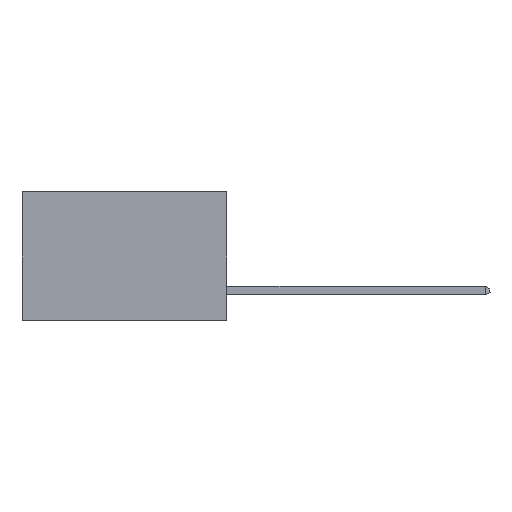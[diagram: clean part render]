
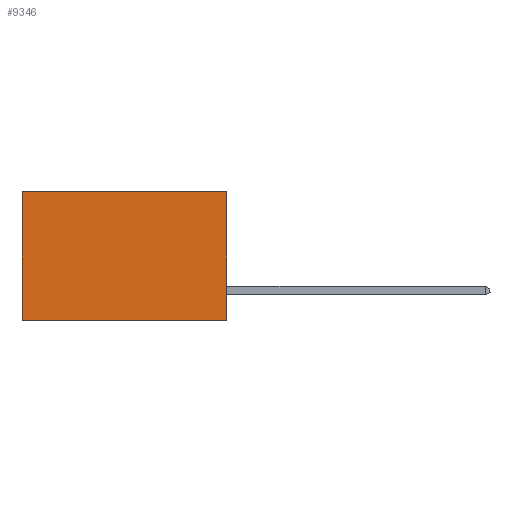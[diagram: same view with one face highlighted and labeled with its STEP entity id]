
A CAD part, left-side view. The second image highlights one B-rep face of the part: STEP entity #9346.
In plain terms, the highlighted planar face has unit normal (-1, 0, 0).
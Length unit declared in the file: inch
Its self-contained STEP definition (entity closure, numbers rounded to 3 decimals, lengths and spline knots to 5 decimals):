
#121 = EDGE_LOOP ( 'NONE', ( #21535, #1404, #6696, #2013 ) ) ;
#1185 = DIRECTION ( 'NONE',  ( 0., 0., -1. ) ) ;
#1189 = DIRECTION ( 'NONE',  ( 1., 0., 0. ) ) ;
#1210 = CARTESIAN_POINT ( 'NONE',  ( 0.277, 0., -0.37 ) ) ;
#1312 = EDGE_CURVE ( 'NONE', #15598, #20218, #22398, .T. ) ;
#1326 = PLANE ( 'NONE',  #8657 ) ;
#1404 = ORIENTED_EDGE ( 'NONE', *, *, #19868, .F. ) ;
#2013 = ORIENTED_EDGE ( 'NONE', *, *, #7317, .T. ) ;
#2120 = CARTESIAN_POINT ( 'NONE',  ( 0.277, 0.59, -0.37 ) ) ;
#2456 = VECTOR ( 'NONE', #13844, 39.37008 ) ;
#4245 = DIRECTION ( 'NONE',  ( 0., 0., -1. ) ) ;
#5901 = CARTESIAN_POINT ( 'NONE',  ( 0.277, 0.59, -0.37 ) ) ;
#6696 = ORIENTED_EDGE ( 'NONE', *, *, #8898, .F. ) ;
#6921 = CARTESIAN_POINT ( 'NONE',  ( 0.277, 0.59, 0. ) ) ;
#7317 = EDGE_CURVE ( 'NONE', #20247, #15598, #17886, .T. ) ;
#8657 = AXIS2_PLACEMENT_3D ( 'NONE', #1210, #1189, #1185 ) ;
#8898 = EDGE_CURVE ( 'NONE', #20247, #12622, #16341, .T. ) ;
#8998 = CARTESIAN_POINT ( 'NONE',  ( 0.277, 0., -0.37 ) ) ;
#9346 = ADVANCED_FACE ( 'NONE', ( #24883 ), #1326, .F. ) ;
#11001 = DIRECTION ( 'NONE',  ( 0., 1., 0. ) ) ;
#12545 = CARTESIAN_POINT ( 'NONE',  ( 0.277, 0., -0.37 ) ) ;
#12622 = VERTEX_POINT ( 'NONE', #12545 ) ;
#12802 = VECTOR ( 'NONE', #14337, 39.37008 ) ;
#13844 = DIRECTION ( 'NONE',  ( 0., 0., -1. ) ) ;
#14337 = DIRECTION ( 'NONE',  ( 0., 1., 0. ) ) ;
#14369 = CARTESIAN_POINT ( 'NONE',  ( 0.277, 0., 0. ) ) ;
#14669 = CARTESIAN_POINT ( 'NONE',  ( 0.277, 0., -0.37 ) ) ;
#15598 = VERTEX_POINT ( 'NONE', #6921 ) ;
#16341 = LINE ( 'NONE', #14669, #2456 ) ;
#17392 = VECTOR ( 'NONE', #4245, 39.37008 ) ;
#17886 = LINE ( 'NONE', #14369, #12802 ) ;
#19868 = EDGE_CURVE ( 'NONE', #12622, #20218, #20036, .T. ) ;
#20036 = LINE ( 'NONE', #8998, #24479 ) ;
#20218 = VERTEX_POINT ( 'NONE', #5901 ) ;
#20247 = VERTEX_POINT ( 'NONE', #23521 ) ;
#21535 = ORIENTED_EDGE ( 'NONE', *, *, #1312, .T. ) ;
#22398 = LINE ( 'NONE', #2120, #17392 ) ;
#23521 = CARTESIAN_POINT ( 'NONE',  ( 0.277, 0., 0. ) ) ;
#24479 = VECTOR ( 'NONE', #11001, 39.37008 ) ;
#24883 = FACE_OUTER_BOUND ( 'NONE', #121, .T. ) ;
